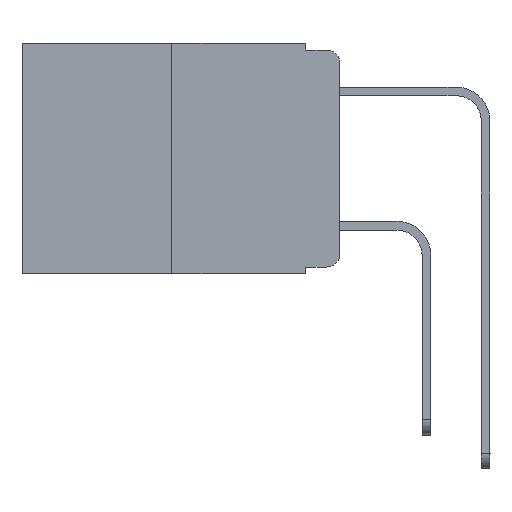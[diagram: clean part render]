
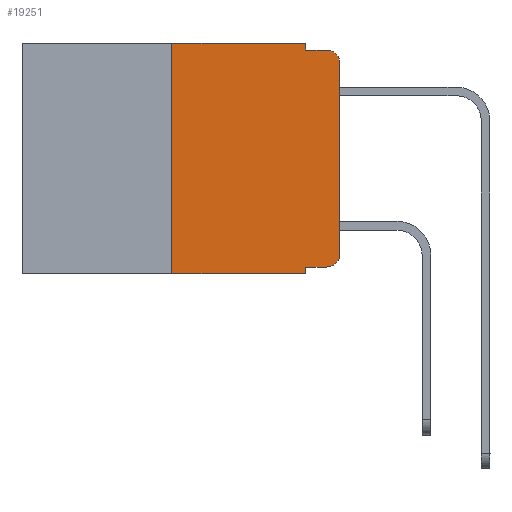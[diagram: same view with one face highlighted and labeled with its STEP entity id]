
A CAD part, left-side view. The second image highlights one B-rep face of the part: STEP entity #19251.
In plain terms, the highlighted planar face has unit normal (-1, 0, 0).
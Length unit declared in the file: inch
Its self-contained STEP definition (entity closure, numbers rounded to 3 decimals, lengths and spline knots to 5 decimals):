
#4 = CARTESIAN_POINT ( 'NONE',  ( 0., 0.051, -0.01 ) ) ;
#907 = DIRECTION ( 'NONE',  ( 0., 0., 1. ) ) ;
#1353 = VERTEX_POINT ( 'NONE', #13309 ) ;
#1488 = CARTESIAN_POINT ( 'NONE',  ( 0., 0.25, 0. ) ) ;
#1638 = LINE ( 'NONE', #5261, #23543 ) ;
#1983 = ORIENTED_EDGE ( 'NONE', *, *, #7535, .F. ) ;
#2301 = LINE ( 'NONE', #21916, #5480 ) ;
#2577 = EDGE_CURVE ( 'NONE', #1353, #24683, #19490, .T. ) ;
#2718 = CARTESIAN_POINT ( 'NONE',  ( 0., 0.02, -0.333 ) ) ;
#2979 = VERTEX_POINT ( 'NONE', #25547 ) ;
#3043 = AXIS2_PLACEMENT_3D ( 'NONE', #19232, #17411, #25536 ) ;
#3847 = VECTOR ( 'NONE', #6707, 39.37008 ) ;
#4030 = DIRECTION ( 'NONE',  ( -1., 0., 0. ) ) ;
#4296 = DIRECTION ( 'NONE',  ( 0., 0., -1. ) ) ;
#4399 = EDGE_CURVE ( 'NONE', #7498, #2979, #23310, .T. ) ;
#4437 = CARTESIAN_POINT ( 'NONE',  ( 0., 0.051, 0. ) ) ;
#4481 = PLANE ( 'NONE',  #3043 ) ;
#4629 = CARTESIAN_POINT ( 'NONE',  ( 0., 0.02, -0.313 ) ) ;
#4678 = VERTEX_POINT ( 'NONE', #17750 ) ;
#4798 = DIRECTION ( 'NONE',  ( 0., 0., -1. ) ) ;
#5261 = CARTESIAN_POINT ( 'NONE',  ( 0., 0.473, 0. ) ) ;
#5480 = VECTOR ( 'NONE', #26271, 39.37008 ) ;
#5932 = ORIENTED_EDGE ( 'NONE', *, *, #17738, .F. ) ;
#6210 = ORIENTED_EDGE ( 'NONE', *, *, #16500, .T. ) ;
#6219 = CIRCLE ( 'NONE', #24137, 0.02 ) ;
#6325 = VERTEX_POINT ( 'NONE', #9601 ) ;
#6337 = DIRECTION ( 'NONE',  ( 0., 0., -1. ) ) ;
#6707 = DIRECTION ( 'NONE',  ( 0., -1., 0. ) ) ;
#6746 = CARTESIAN_POINT ( 'NONE',  ( 0., 0.473, -0.343 ) ) ;
#7498 = VERTEX_POINT ( 'NONE', #16516 ) ;
#7500 = DIRECTION ( 'NONE',  ( 0., 0., 1. ) ) ;
#7535 = EDGE_CURVE ( 'NONE', #19953, #21419, #1638, .T. ) ;
#7622 = ORIENTED_EDGE ( 'NONE', *, *, #19794, .T. ) ;
#8752 = VECTOR ( 'NONE', #4798, 39.37008 ) ;
#9118 = EDGE_CURVE ( 'NONE', #21419, #12820, #11559, .T. ) ;
#9601 = CARTESIAN_POINT ( 'NONE',  ( 0., 0.02, -0.01 ) ) ;
#10721 = CIRCLE ( 'NONE', #11636, 0.02 ) ;
#10851 = EDGE_CURVE ( 'NONE', #7498, #19953, #25024, .T. ) ;
#11559 = LINE ( 'NONE', #17745, #8752 ) ;
#11636 = AXIS2_PLACEMENT_3D ( 'NONE', #4629, #19528, #6337 ) ;
#12192 = VECTOR ( 'NONE', #7500, 39.37008 ) ;
#12597 = CARTESIAN_POINT ( 'NONE',  ( 0., 0.051, 0. ) ) ;
#12624 = DIRECTION ( 'NONE',  ( 0., 0., -1. ) ) ;
#12820 = VERTEX_POINT ( 'NONE', #4 ) ;
#13309 = CARTESIAN_POINT ( 'NONE',  ( 0., 0.051, -0.333 ) ) ;
#13326 = VECTOR ( 'NONE', #907, 39.37008 ) ;
#13418 = CARTESIAN_POINT ( 'NONE',  ( 0., 0., 0. ) ) ;
#13427 = CARTESIAN_POINT ( 'NONE',  ( 0., 0.25, 0. ) ) ;
#13604 = ORIENTED_EDGE ( 'NONE', *, *, #4399, .T. ) ;
#13832 = DIRECTION ( 'NONE',  ( 0., -1., 0. ) ) ;
#14349 = EDGE_CURVE ( 'NONE', #24683, #4678, #10721, .T. ) ;
#15106 = LINE ( 'NONE', #13418, #12192 ) ;
#15185 = ORIENTED_EDGE ( 'NONE', *, *, #14349, .T. ) ;
#15585 = VERTEX_POINT ( 'NONE', #26109 ) ;
#16500 = EDGE_CURVE ( 'NONE', #4678, #15585, #15106, .T. ) ;
#16516 = CARTESIAN_POINT ( 'NONE',  ( 0., 0.25, -0.343 ) ) ;
#17095 = LINE ( 'NONE', #4437, #26763 ) ;
#17139 = FACE_OUTER_BOUND ( 'NONE', #19329, .T. ) ;
#17153 = DIRECTION ( 'NONE',  ( 0., -1., 0. ) ) ;
#17411 = DIRECTION ( 'NONE',  ( 1., 0., 0. ) ) ;
#17652 = ORIENTED_EDGE ( 'NONE', *, *, #9118, .F. ) ;
#17693 = VECTOR ( 'NONE', #17153, 39.37008 ) ;
#17738 = EDGE_CURVE ( 'NONE', #1353, #2979, #17095, .T. ) ;
#17745 = CARTESIAN_POINT ( 'NONE',  ( 0., 0.051, 0. ) ) ;
#17750 = CARTESIAN_POINT ( 'NONE',  ( 0., 0., -0.313 ) ) ;
#18883 = ORIENTED_EDGE ( 'NONE', *, *, #10851, .F. ) ;
#19232 = CARTESIAN_POINT ( 'NONE',  ( 0., 0.473, 0. ) ) ;
#19251 = ADVANCED_FACE ( 'NONE', ( #17139 ), #4481, .F. ) ;
#19329 = EDGE_LOOP ( 'NONE', ( #6210, #7622, #24384, #17652, #1983, #18883, #13604, #5932, #27568, #15185 ) ) ;
#19490 = LINE ( 'NONE', #21576, #3847 ) ;
#19528 = DIRECTION ( 'NONE',  ( -1., 0., 0. ) ) ;
#19794 = EDGE_CURVE ( 'NONE', #15585, #6325, #6219, .T. ) ;
#19953 = VERTEX_POINT ( 'NONE', #13427 ) ;
#21419 = VERTEX_POINT ( 'NONE', #12597 ) ;
#21576 = CARTESIAN_POINT ( 'NONE',  ( 0., 0.051, -0.333 ) ) ;
#21916 = CARTESIAN_POINT ( 'NONE',  ( 0., 0.051, -0.01 ) ) ;
#23310 = LINE ( 'NONE', #6746, #17693 ) ;
#23543 = VECTOR ( 'NONE', #13832, 39.37008 ) ;
#24137 = AXIS2_PLACEMENT_3D ( 'NONE', #25779, #4030, #12624 ) ;
#24384 = ORIENTED_EDGE ( 'NONE', *, *, #24691, .F. ) ;
#24683 = VERTEX_POINT ( 'NONE', #2718 ) ;
#24691 = EDGE_CURVE ( 'NONE', #12820, #6325, #2301, .T. ) ;
#25024 = LINE ( 'NONE', #1488, #13326 ) ;
#25536 = DIRECTION ( 'NONE',  ( 0., 0., -1. ) ) ;
#25547 = CARTESIAN_POINT ( 'NONE',  ( 0., 0.051, -0.343 ) ) ;
#25779 = CARTESIAN_POINT ( 'NONE',  ( 0., 0.02, -0.03 ) ) ;
#26109 = CARTESIAN_POINT ( 'NONE',  ( 0., 0., -0.03 ) ) ;
#26271 = DIRECTION ( 'NONE',  ( 0., -1., 0. ) ) ;
#26763 = VECTOR ( 'NONE', #4296, 39.37008 ) ;
#27568 = ORIENTED_EDGE ( 'NONE', *, *, #2577, .T. ) ;
